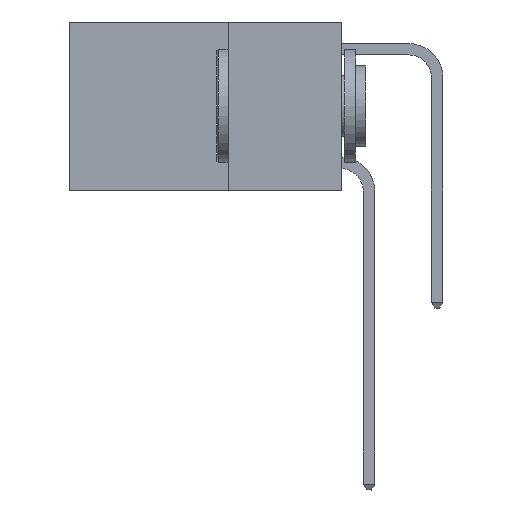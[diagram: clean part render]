
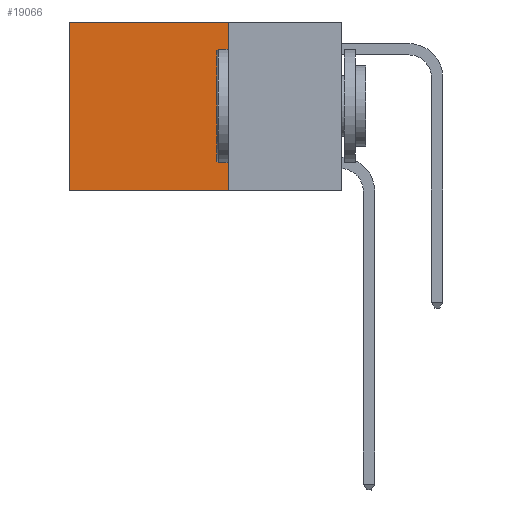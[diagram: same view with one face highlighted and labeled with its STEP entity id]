
A CAD part, left-side view. The second image highlights one B-rep face of the part: STEP entity #19066.
In plain terms, the highlighted planar face has unit normal (-1, 0, 0).
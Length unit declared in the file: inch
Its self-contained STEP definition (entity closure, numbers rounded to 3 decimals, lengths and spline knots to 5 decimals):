
#3084 = PLANE ( 'NONE',  #3598 ) ;
#3186 = DIRECTION ( 'NONE',  ( 0., 0., -1. ) ) ;
#3469 = VECTOR ( 'NONE', #19812, 39.37008 ) ;
#3598 = AXIS2_PLACEMENT_3D ( 'NONE', #10479, #29910, #3186 ) ;
#5657 = CARTESIAN_POINT ( 'NONE',  ( 0.2625, 0.6, 0. ) ) ;
#6664 = CARTESIAN_POINT ( 'NONE',  ( 0.2625, 0.25, -0.37 ) ) ;
#8197 = CARTESIAN_POINT ( 'NONE',  ( 0.2625, 0.25, 0. ) ) ;
#8749 = ORIENTED_EDGE ( 'NONE', *, *, #28897, .F. ) ;
#10479 = CARTESIAN_POINT ( 'NONE',  ( 0.2625, 0.25, 0. ) ) ;
#10942 = VECTOR ( 'NONE', #16726, 39.37008 ) ;
#11265 = CARTESIAN_POINT ( 'NONE',  ( 0.2625, 0.6, -0.37 ) ) ;
#11294 = VERTEX_POINT ( 'NONE', #8197 ) ;
#11398 = LINE ( 'NONE', #5657, #3469 ) ;
#11721 = LINE ( 'NONE', #15957, #23889 ) ;
#12445 = ORIENTED_EDGE ( 'NONE', *, *, #13395, .F. ) ;
#13395 = EDGE_CURVE ( 'NONE', #11294, #17729, #11721, .T. ) ;
#13642 = VERTEX_POINT ( 'NONE', #23675 ) ;
#13680 = ORIENTED_EDGE ( 'NONE', *, *, #19504, .T. ) ;
#14085 = FACE_OUTER_BOUND ( 'NONE', #30601, .T. ) ;
#15957 = CARTESIAN_POINT ( 'NONE',  ( 0.2625, 0.25, 0. ) ) ;
#16726 = DIRECTION ( 'NONE',  ( 0., 1., 0. ) ) ;
#17328 = ORIENTED_EDGE ( 'NONE', *, *, #30710, .T. ) ;
#17729 = VERTEX_POINT ( 'NONE', #6664 ) ;
#19066 = ADVANCED_FACE ( 'NONE', ( #14085 ), #3084, .F. ) ;
#19504 = EDGE_CURVE ( 'NONE', #13642, #20795, #11398, .T. ) ;
#19812 = DIRECTION ( 'NONE',  ( 0., 0., -1. ) ) ;
#20495 = LINE ( 'NONE', #21184, #28529 ) ;
#20795 = VERTEX_POINT ( 'NONE', #11265 ) ;
#21184 = CARTESIAN_POINT ( 'NONE',  ( 0.2625, 0.25, -0.37 ) ) ;
#23675 = CARTESIAN_POINT ( 'NONE',  ( 0.2625, 0.6, 0. ) ) ;
#23889 = VECTOR ( 'NONE', #25442, 39.37008 ) ;
#25442 = DIRECTION ( 'NONE',  ( 0., 0., -1. ) ) ;
#28467 = LINE ( 'NONE', #31428, #10942 ) ;
#28529 = VECTOR ( 'NONE', #28696, 39.37008 ) ;
#28696 = DIRECTION ( 'NONE',  ( 0., 1., 0. ) ) ;
#28897 = EDGE_CURVE ( 'NONE', #17729, #20795, #20495, .T. ) ;
#29910 = DIRECTION ( 'NONE',  ( 1., 0., 0. ) ) ;
#30601 = EDGE_LOOP ( 'NONE', ( #13680, #8749, #12445, #17328 ) ) ;
#30710 = EDGE_CURVE ( 'NONE', #11294, #13642, #28467, .T. ) ;
#31428 = CARTESIAN_POINT ( 'NONE',  ( 0.2625, 0.25, 0. ) ) ;
